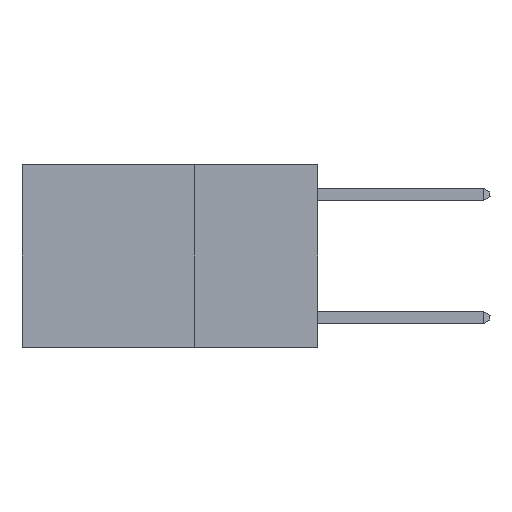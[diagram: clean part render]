
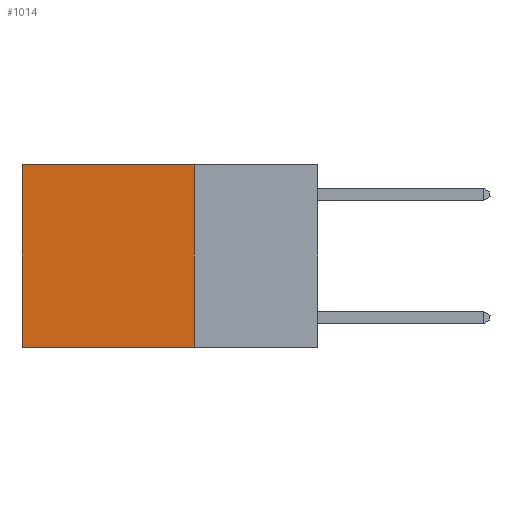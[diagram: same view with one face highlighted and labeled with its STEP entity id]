
A CAD part, left-side view. The second image highlights one B-rep face of the part: STEP entity #1014.
In plain terms, the highlighted planar face has unit normal (-1, 0, 0).
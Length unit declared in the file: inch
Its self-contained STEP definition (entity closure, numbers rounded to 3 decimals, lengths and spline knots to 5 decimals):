
#29 = LINE ( 'NONE', #3595, #5324 ) ;
#136 = DIRECTION ( 'NONE',  ( 0., 1., 0. ) ) ;
#342 = ORIENTED_EDGE ( 'NONE', *, *, #12464, .F. ) ;
#754 = DIRECTION ( 'NONE',  ( 0., 0., -1. ) ) ;
#1014 = ADVANCED_FACE ( 'NONE', ( #6331 ), #10897, .F. ) ;
#1151 = CARTESIAN_POINT ( 'NONE',  ( 0.2625, 0.25, 0. ) ) ;
#1202 = ORIENTED_EDGE ( 'NONE', *, *, #13224, .F. ) ;
#1260 = CARTESIAN_POINT ( 'NONE',  ( 0.2625, 0.25, -0.37 ) ) ;
#1911 = AXIS2_PLACEMENT_3D ( 'NONE', #12167, #12096, #754 ) ;
#1989 = LINE ( 'NONE', #12416, #14235 ) ;
#2032 = CARTESIAN_POINT ( 'NONE',  ( 0.2625, 0.6, -0.37 ) ) ;
#2571 = VERTEX_POINT ( 'NONE', #13084 ) ;
#2920 = EDGE_CURVE ( 'NONE', #2571, #5049, #1989, .T. ) ;
#3595 = CARTESIAN_POINT ( 'NONE',  ( 0.2625, 0.25, 0. ) ) ;
#4760 = DIRECTION ( 'NONE',  ( 0., 1., 0. ) ) ;
#5049 = VERTEX_POINT ( 'NONE', #2032 ) ;
#5324 = VECTOR ( 'NONE', #4760, 39.37008 ) ;
#5664 = EDGE_LOOP ( 'NONE', ( #12050, #342, #1202, #12119 ) ) ;
#6037 = VECTOR ( 'NONE', #136, 39.37008 ) ;
#6331 = FACE_OUTER_BOUND ( 'NONE', #5664, .T. ) ;
#7056 = LINE ( 'NONE', #1260, #6037 ) ;
#7905 = CARTESIAN_POINT ( 'NONE',  ( 0.2625, 0.25, 0. ) ) ;
#8692 = VECTOR ( 'NONE', #11654, 39.37008 ) ;
#8971 = DIRECTION ( 'NONE',  ( 0., 0., -1. ) ) ;
#9212 = VERTEX_POINT ( 'NONE', #7905 ) ;
#10897 = PLANE ( 'NONE',  #1911 ) ;
#11654 = DIRECTION ( 'NONE',  ( 0., 0., -1. ) ) ;
#11812 = LINE ( 'NONE', #1151, #8692 ) ;
#11823 = VERTEX_POINT ( 'NONE', #12764 ) ;
#12050 = ORIENTED_EDGE ( 'NONE', *, *, #2920, .T. ) ;
#12096 = DIRECTION ( 'NONE',  ( 1., 0., 0. ) ) ;
#12119 = ORIENTED_EDGE ( 'NONE', *, *, #13180, .T. ) ;
#12167 = CARTESIAN_POINT ( 'NONE',  ( 0.2625, 0.25, 0. ) ) ;
#12416 = CARTESIAN_POINT ( 'NONE',  ( 0.2625, 0.6, 0. ) ) ;
#12464 = EDGE_CURVE ( 'NONE', #11823, #5049, #7056, .T. ) ;
#12764 = CARTESIAN_POINT ( 'NONE',  ( 0.2625, 0.25, -0.37 ) ) ;
#13084 = CARTESIAN_POINT ( 'NONE',  ( 0.2625, 0.6, 0. ) ) ;
#13180 = EDGE_CURVE ( 'NONE', #9212, #2571, #29, .T. ) ;
#13224 = EDGE_CURVE ( 'NONE', #9212, #11823, #11812, .T. ) ;
#14235 = VECTOR ( 'NONE', #8971, 39.37008 ) ;
